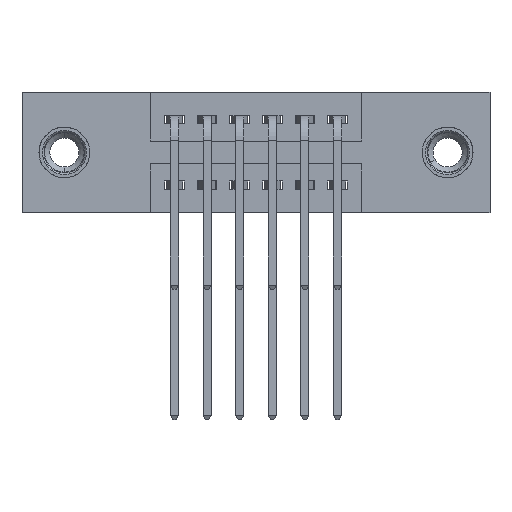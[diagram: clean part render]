
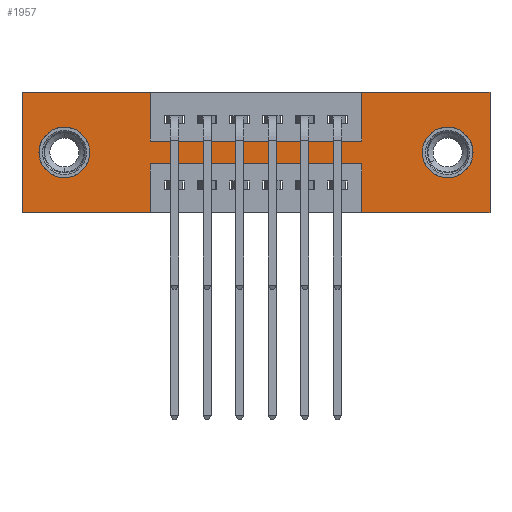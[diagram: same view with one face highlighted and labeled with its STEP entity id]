
A CAD part, front view. The second image highlights one B-rep face of the part: STEP entity #1957.
In plain terms, the highlighted planar face has unit normal (0, -1, 0).
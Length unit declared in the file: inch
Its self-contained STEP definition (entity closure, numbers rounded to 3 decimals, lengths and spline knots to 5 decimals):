
#166 = LINE ( 'NONE', #532, #6322 ) ;
#210 = VECTOR ( 'NONE', #11964, 39.37008 ) ;
#237 = EDGE_CURVE ( 'NONE', #8681, #11067, #12272, .T. ) ;
#488 = AXIS2_PLACEMENT_3D ( 'NONE', #3895, #7793, #6870 ) ;
#524 = VERTEX_POINT ( 'NONE', #5016 ) ;
#532 = CARTESIAN_POINT ( 'NONE',  ( 1.0425, 0., -0.37 ) ) ;
#613 = DIRECTION ( 'NONE',  ( 0., 1., 0. ) ) ;
#620 = VERTEX_POINT ( 'NONE', #8035 ) ;
#687 = LINE ( 'NONE', #11177, #5519 ) ;
#746 = DIRECTION ( 'NONE',  ( -1., 0., 0. ) ) ;
#811 = ORIENTED_EDGE ( 'NONE', *, *, #11512, .F. ) ;
#847 = LINE ( 'NONE', #7300, #2661 ) ;
#854 = AXIS2_PLACEMENT_3D ( 'NONE', #10195, #9274, #2474 ) ;
#955 = CARTESIAN_POINT ( 'NONE',  ( 0., 0., -0.37 ) ) ;
#1139 = CARTESIAN_POINT ( 'NONE',  ( 1.305, 0., -0.185 ) ) ;
#1310 = VERTEX_POINT ( 'NONE', #9770 ) ;
#1382 = EDGE_LOOP ( 'NONE', ( #4678, #811, #2749, #6194, #3089, #6245, #8039, #2593, #7264, #6626, #4936, #1487 ) ) ;
#1487 = ORIENTED_EDGE ( 'NONE', *, *, #6060, .F. ) ;
#1586 = DIRECTION ( 'NONE',  ( 0., 0., -1. ) ) ;
#1871 = VERTEX_POINT ( 'NONE', #8572 ) ;
#1957 = ADVANCED_FACE ( 'NONE', ( #3450, #5251, #9677 ), #7254, .T. ) ;
#1958 = VECTOR ( 'NONE', #11724, 39.37008 ) ;
#1997 = DIRECTION ( 'NONE',  ( 1., 0., 0. ) ) ;
#2067 = CARTESIAN_POINT ( 'NONE',  ( 0., 0., -0.37 ) ) ;
#2173 = LINE ( 'NONE', #7849, #9355 ) ;
#2257 = VECTOR ( 'NONE', #3678, 39.37008 ) ;
#2474 = DIRECTION ( 'NONE',  ( 0., 0., 1. ) ) ;
#2531 = CARTESIAN_POINT ( 'NONE',  ( 0., 0., -0.37 ) ) ;
#2561 = CARTESIAN_POINT ( 'NONE',  ( 0.13, 0., -0.107 ) ) ;
#2593 = ORIENTED_EDGE ( 'NONE', *, *, #8275, .F. ) ;
#2639 = LINE ( 'NONE', #6461, #6972 ) ;
#2656 = CARTESIAN_POINT ( 'NONE',  ( 1.0425, 0., -0.22 ) ) ;
#2661 = VECTOR ( 'NONE', #746, 39.37008 ) ;
#2693 = CARTESIAN_POINT ( 'NONE',  ( 0.13, 0., -0.263 ) ) ;
#2749 = ORIENTED_EDGE ( 'NONE', *, *, #7297, .F. ) ;
#3000 = CARTESIAN_POINT ( 'NONE',  ( 0., 0., 0. ) ) ;
#3089 = ORIENTED_EDGE ( 'NONE', *, *, #6981, .F. ) ;
#3191 = EDGE_LOOP ( 'NONE', ( #11834, #5447 ) ) ;
#3240 = VECTOR ( 'NONE', #1997, 39.37008 ) ;
#3450 = FACE_BOUND ( 'NONE', #3191, .T. ) ;
#3513 = DIRECTION ( 'NONE',  ( 0., 0., -1. ) ) ;
#3678 = DIRECTION ( 'NONE',  ( -1., 0., 0. ) ) ;
#3715 = AXIS2_PLACEMENT_3D ( 'NONE', #2531, #5512, #3513 ) ;
#3895 = CARTESIAN_POINT ( 'NONE',  ( 1.305, 0., -0.185 ) ) ;
#4132 = EDGE_CURVE ( 'NONE', #5716, #524, #2173, .T. ) ;
#4137 = CIRCLE ( 'NONE', #11526, 0.078 ) ;
#4152 = EDGE_CURVE ( 'NONE', #7340, #7011, #2639, .T. ) ;
#4402 = DIRECTION ( 'NONE',  ( 0., 0., 1. ) ) ;
#4456 = AXIS2_PLACEMENT_3D ( 'NONE', #6374, #613, #7326 ) ;
#4678 = ORIENTED_EDGE ( 'NONE', *, *, #4132, .F. ) ;
#4681 = CARTESIAN_POINT ( 'NONE',  ( 0., 0., -0.37 ) ) ;
#4769 = EDGE_CURVE ( 'NONE', #9306, #620, #9196, .T. ) ;
#4936 = ORIENTED_EDGE ( 'NONE', *, *, #11590, .F. ) ;
#4992 = CARTESIAN_POINT ( 'NONE',  ( 0.3925, 0., -0.15 ) ) ;
#5016 = CARTESIAN_POINT ( 'NONE',  ( 0.3925, 0., -0.37 ) ) ;
#5090 = ORIENTED_EDGE ( 'NONE', *, *, #6969, .T. ) ;
#5206 = DIRECTION ( 'NONE',  ( 1., 0., 0. ) ) ;
#5251 = FACE_BOUND ( 'NONE', #6487, .T. ) ;
#5447 = ORIENTED_EDGE ( 'NONE', *, *, #9653, .T. ) ;
#5512 = DIRECTION ( 'NONE',  ( 0., -1., 0. ) ) ;
#5519 = VECTOR ( 'NONE', #6381, 39.37008 ) ;
#5701 = VECTOR ( 'NONE', #5206, 39.37008 ) ;
#5716 = VERTEX_POINT ( 'NONE', #9341 ) ;
#5999 = LINE ( 'NONE', #3000, #11346 ) ;
#6060 = EDGE_CURVE ( 'NONE', #524, #8712, #12139, .T. ) ;
#6164 = LINE ( 'NONE', #955, #2257 ) ;
#6194 = ORIENTED_EDGE ( 'NONE', *, *, #8125, .F. ) ;
#6233 = CARTESIAN_POINT ( 'NONE',  ( 0., 0., 0. ) ) ;
#6241 = CARTESIAN_POINT ( 'NONE',  ( 1.0425, 0., -0.15 ) ) ;
#6245 = ORIENTED_EDGE ( 'NONE', *, *, #10192, .F. ) ;
#6256 = CARTESIAN_POINT ( 'NONE',  ( 0.3925, 0., 0. ) ) ;
#6322 = VECTOR ( 'NONE', #4402, 39.37008 ) ;
#6374 = CARTESIAN_POINT ( 'NONE',  ( 0.13, 0., -0.185 ) ) ;
#6381 = DIRECTION ( 'NONE',  ( 0., 0., 1. ) ) ;
#6461 = CARTESIAN_POINT ( 'NONE',  ( 0.3925, 0., 0. ) ) ;
#6487 = EDGE_LOOP ( 'NONE', ( #10467, #5090 ) ) ;
#6626 = ORIENTED_EDGE ( 'NONE', *, *, #10627, .F. ) ;
#6736 = VERTEX_POINT ( 'NONE', #7004 ) ;
#6768 = CARTESIAN_POINT ( 'NONE',  ( 1.0425, 0., -0.37 ) ) ;
#6870 = DIRECTION ( 'NONE',  ( 0., 0., -1. ) ) ;
#6969 = EDGE_CURVE ( 'NONE', #11067, #8681, #10497, .T. ) ;
#6972 = VECTOR ( 'NONE', #12039, 39.37008 ) ;
#6981 = EDGE_CURVE ( 'NONE', #10385, #1871, #11696, .T. ) ;
#7004 = CARTESIAN_POINT ( 'NONE',  ( 0., 0., 0. ) ) ;
#7011 = VERTEX_POINT ( 'NONE', #9483 ) ;
#7254 = PLANE ( 'NONE',  #3715 ) ;
#7264 = ORIENTED_EDGE ( 'NONE', *, *, #4152, .F. ) ;
#7297 = EDGE_CURVE ( 'NONE', #7740, #9854, #166, .T. ) ;
#7300 = CARTESIAN_POINT ( 'NONE',  ( 0.3925, 0., -0.22 ) ) ;
#7326 = DIRECTION ( 'NONE',  ( 0., 0., 1. ) ) ;
#7340 = VERTEX_POINT ( 'NONE', #6256 ) ;
#7740 = VERTEX_POINT ( 'NONE', #6768 ) ;
#7793 = DIRECTION ( 'NONE',  ( 0., 1., 0. ) ) ;
#7846 = DIRECTION ( 'NONE',  ( 0., 1., 0. ) ) ;
#7849 = CARTESIAN_POINT ( 'NONE',  ( 0.3925, 0., -0.37 ) ) ;
#8035 = CARTESIAN_POINT ( 'NONE',  ( 1.0425, 0., 0. ) ) ;
#8039 = ORIENTED_EDGE ( 'NONE', *, *, #4769, .F. ) ;
#8125 = EDGE_CURVE ( 'NONE', #1871, #7740, #6164, .T. ) ;
#8275 = EDGE_CURVE ( 'NONE', #7011, #9306, #8594, .T. ) ;
#8572 = CARTESIAN_POINT ( 'NONE',  ( 1.435, 0., -0.37 ) ) ;
#8583 = DIRECTION ( 'NONE',  ( 1., 0., 0. ) ) ;
#8594 = LINE ( 'NONE', #4992, #3240 ) ;
#8669 = LINE ( 'NONE', #6233, #5701 ) ;
#8681 = VERTEX_POINT ( 'NONE', #2561 ) ;
#8712 = VERTEX_POINT ( 'NONE', #4681 ) ;
#9142 = DIRECTION ( 'NONE',  ( 0., 0., -1. ) ) ;
#9196 = LINE ( 'NONE', #10053, #210 ) ;
#9274 = DIRECTION ( 'NONE',  ( 0., 1., 0. ) ) ;
#9306 = VERTEX_POINT ( 'NONE', #6241 ) ;
#9341 = CARTESIAN_POINT ( 'NONE',  ( 0.3925, 0., -0.22 ) ) ;
#9355 = VECTOR ( 'NONE', #9142, 39.37008 ) ;
#9483 = CARTESIAN_POINT ( 'NONE',  ( 0.3925, 0., -0.15 ) ) ;
#9653 = EDGE_CURVE ( 'NONE', #10250, #1310, #4137, .T. ) ;
#9677 = FACE_OUTER_BOUND ( 'NONE', #1382, .T. ) ;
#9754 = DIRECTION ( 'NONE',  ( 0., 0., -1. ) ) ;
#9770 = CARTESIAN_POINT ( 'NONE',  ( 1.305, 0., -0.107 ) ) ;
#9854 = VERTEX_POINT ( 'NONE', #2656 ) ;
#9885 = CARTESIAN_POINT ( 'NONE',  ( 1.305, 0., -0.263 ) ) ;
#10053 = CARTESIAN_POINT ( 'NONE',  ( 1.0425, 0., 0. ) ) ;
#10192 = EDGE_CURVE ( 'NONE', #620, #10385, #8669, .T. ) ;
#10195 = CARTESIAN_POINT ( 'NONE',  ( 0.13, 0., -0.185 ) ) ;
#10204 = CARTESIAN_POINT ( 'NONE',  ( 1.435, 0., 0. ) ) ;
#10250 = VERTEX_POINT ( 'NONE', #9885 ) ;
#10385 = VERTEX_POINT ( 'NONE', #12126 ) ;
#10467 = ORIENTED_EDGE ( 'NONE', *, *, #237, .T. ) ;
#10497 = CIRCLE ( 'NONE', #4456, 0.078 ) ;
#10592 = EDGE_CURVE ( 'NONE', #1310, #10250, #12396, .T. ) ;
#10627 = EDGE_CURVE ( 'NONE', #6736, #7340, #5999, .T. ) ;
#10803 = VECTOR ( 'NONE', #1586, 39.37008 ) ;
#11067 = VERTEX_POINT ( 'NONE', #2693 ) ;
#11177 = CARTESIAN_POINT ( 'NONE',  ( 0., 0., 0. ) ) ;
#11346 = VECTOR ( 'NONE', #8583, 39.37008 ) ;
#11512 = EDGE_CURVE ( 'NONE', #9854, #5716, #847, .T. ) ;
#11526 = AXIS2_PLACEMENT_3D ( 'NONE', #1139, #7846, #9754 ) ;
#11590 = EDGE_CURVE ( 'NONE', #8712, #6736, #687, .T. ) ;
#11696 = LINE ( 'NONE', #10204, #10803 ) ;
#11724 = DIRECTION ( 'NONE',  ( -1., 0., 0. ) ) ;
#11834 = ORIENTED_EDGE ( 'NONE', *, *, #10592, .T. ) ;
#11964 = DIRECTION ( 'NONE',  ( 0., 0., 1. ) ) ;
#12039 = DIRECTION ( 'NONE',  ( 0., 0., -1. ) ) ;
#12126 = CARTESIAN_POINT ( 'NONE',  ( 1.435, 0., 0. ) ) ;
#12139 = LINE ( 'NONE', #2067, #1958 ) ;
#12272 = CIRCLE ( 'NONE', #854, 0.078 ) ;
#12396 = CIRCLE ( 'NONE', #488, 0.078 ) ;
